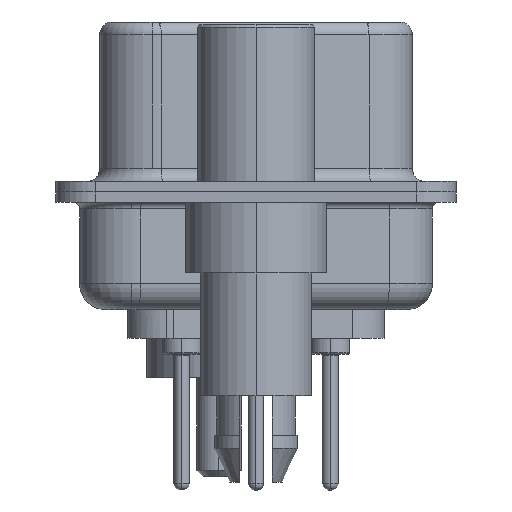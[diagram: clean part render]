
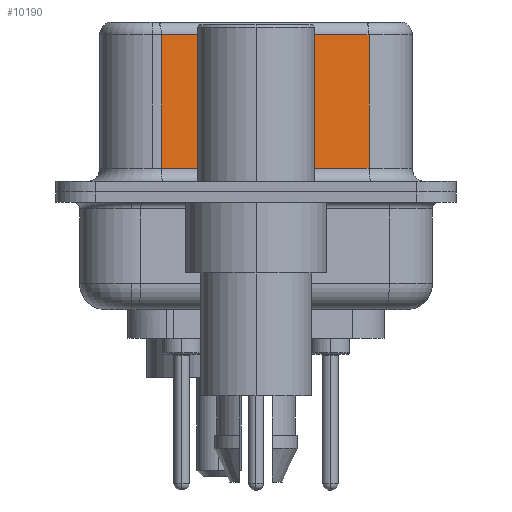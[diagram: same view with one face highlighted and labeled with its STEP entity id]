
A CAD part, left-side view. The second image highlights one B-rep face of the part: STEP entity #10190.
In plain terms, the highlighted planar face has unit normal (-0.985, -0.174, 0).
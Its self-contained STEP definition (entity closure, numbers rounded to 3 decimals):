
#560 = CARTESIAN_POINT ( 'NONE',  ( 5.132, -4.322, 6.02 ) ) ;
#1781 = EDGE_LOOP ( 'NONE', ( #5519, #17015, #25456, #27136 ) ) ;
#1804 = DIRECTION ( 'NONE',  ( 0.985, 0.174, 0. ) ) ;
#1831 = VERTEX_POINT ( 'NONE', #27057 ) ;
#2188 = AXIS2_PLACEMENT_3D ( 'NONE', #13297, #1804, #17996 ) ;
#3141 = CARTESIAN_POINT ( 'NONE',  ( 3.73, 3.628, 6.02 ) ) ;
#3857 = CARTESIAN_POINT ( 'NONE',  ( 5.132, -4.322, 0.9 ) ) ;
#4196 = CARTESIAN_POINT ( 'NONE',  ( 3.73, 3.628, 6.52 ) ) ;
#4264 = LINE ( 'NONE', #4196, #12512 ) ;
#4675 = LINE ( 'NONE', #560, #24450 ) ;
#5519 = ORIENTED_EDGE ( 'NONE', *, *, #24241, .F. ) ;
#5802 = VECTOR ( 'NONE', #5892, 1000. ) ;
#5892 = DIRECTION ( 'NONE',  ( 0.174, -0.985, 0. ) ) ;
#6212 = VERTEX_POINT ( 'NONE', #3141 ) ;
#9009 = EDGE_CURVE ( 'NONE', #1831, #6212, #4675, .T. ) ;
#9218 = VERTEX_POINT ( 'NONE', #3857 ) ;
#9918 = EDGE_CURVE ( 'NONE', #6212, #28615, #4264, .T. ) ;
#10190 = ADVANCED_FACE ( 'NONE', ( #26946 ), #15493, .F. ) ;
#12512 = VECTOR ( 'NONE', #20355, 1000. ) ;
#12598 = CARTESIAN_POINT ( 'NONE',  ( 5.132, -4.322, 0.9 ) ) ;
#13297 = CARTESIAN_POINT ( 'NONE',  ( 5.132, -4.322, 6.52 ) ) ;
#13858 = CARTESIAN_POINT ( 'NONE',  ( 5.132, -4.322, 6.52 ) ) ;
#14121 = VECTOR ( 'NONE', #27609, 1000. ) ;
#15493 = PLANE ( 'NONE',  #2188 ) ;
#17015 = ORIENTED_EDGE ( 'NONE', *, *, #9009, .T. ) ;
#17396 = CARTESIAN_POINT ( 'NONE',  ( 3.73, 3.628, 0.9 ) ) ;
#17992 = LINE ( 'NONE', #12598, #5802 ) ;
#17996 = DIRECTION ( 'NONE',  ( -0.174, 0.985, 0. ) ) ;
#18986 = DIRECTION ( 'NONE',  ( -0.174, 0.985, 0. ) ) ;
#20355 = DIRECTION ( 'NONE',  ( 0., 0., -1. ) ) ;
#24241 = EDGE_CURVE ( 'NONE', #1831, #9218, #24945, .T. ) ;
#24450 = VECTOR ( 'NONE', #18986, 1000. ) ;
#24945 = LINE ( 'NONE', #13858, #14121 ) ;
#25456 = ORIENTED_EDGE ( 'NONE', *, *, #9918, .T. ) ;
#25614 = EDGE_CURVE ( 'NONE', #28615, #9218, #17992, .T. ) ;
#26946 = FACE_OUTER_BOUND ( 'NONE', #1781, .T. ) ;
#27057 = CARTESIAN_POINT ( 'NONE',  ( 5.132, -4.322, 6.02 ) ) ;
#27136 = ORIENTED_EDGE ( 'NONE', *, *, #25614, .T. ) ;
#27609 = DIRECTION ( 'NONE',  ( 0., 0., -1. ) ) ;
#28615 = VERTEX_POINT ( 'NONE', #17396 ) ;
